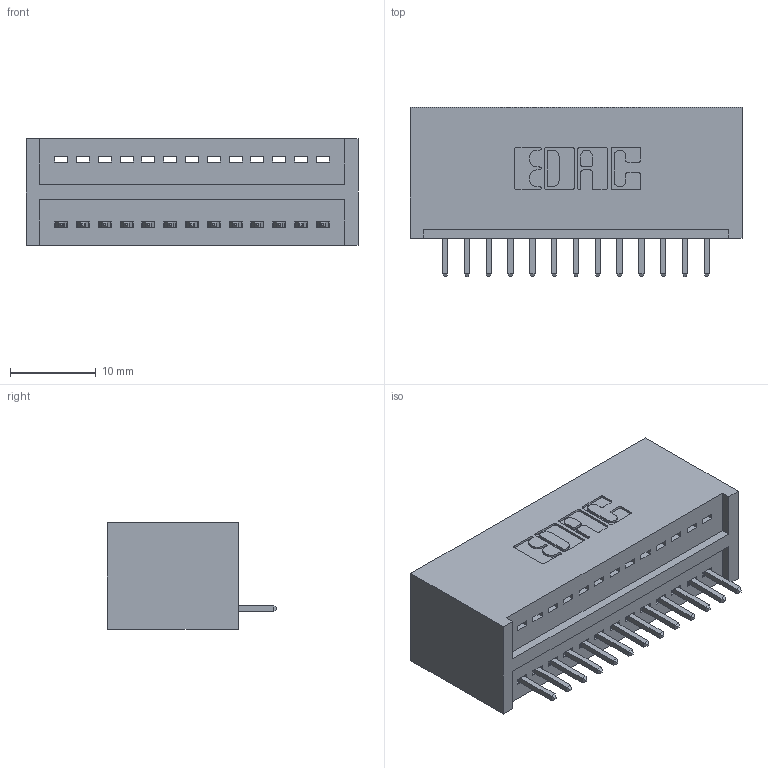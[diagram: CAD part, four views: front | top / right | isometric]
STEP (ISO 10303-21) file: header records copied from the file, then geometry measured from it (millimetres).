
FILE_DESCRIPTION (( 'STEP AP203' ), '1' );
FILE_NAME ('325-013-520-101.STEP', '2020-02-24T15:40:16', ( '' ), ( '' ), 'SwSTEP 2.0', 'SolidWorks 2016', '' );
FILE_SCHEMA (( 'CONFIG_CONTROL_DESIGN' ));
Length unit declared in the file: inch
Products named in the file (3): 325 Part_Lugless; 325-292-001_325-293-120; 325-013-520-101
Assembly tree (14 placements, depth 2):
  325-013-520-101
    325 Part_Lugless
    325-292-001_325-293-120  x13
Bounding box: 38.66 x 19.68 x 12.45 mm (x, y, z)
Volume: 5217.7 mm3; surface area: 5562.1 mm2
Topology: 14 solids, 14 shells, 860 faces, 2575 edges, 1698 vertices
Faces by surface type: plane 612, cylinder 248
Entity records: 11439 total; most frequent: CARTESIAN_POINT 1985, ORIENTED_EDGE 1934, DIRECTION 1725, EDGE_CURVE 967, VECTOR 847, LINE 847, VERTEX_POINT 642, AXIS2_PLACEMENT_3D 439
